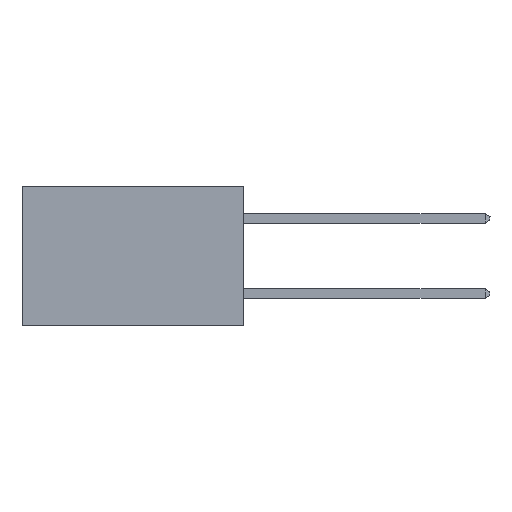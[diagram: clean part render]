
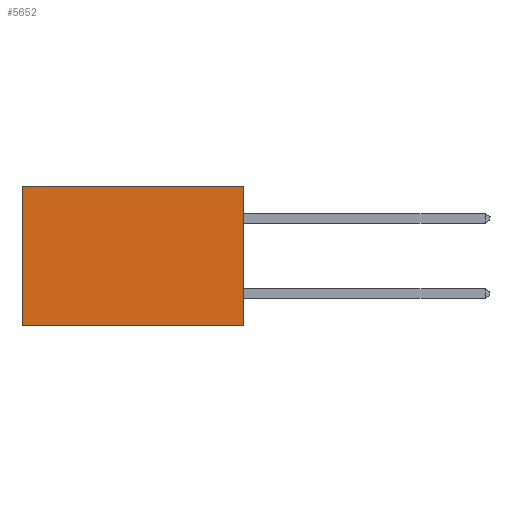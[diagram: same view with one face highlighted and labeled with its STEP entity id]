
A CAD part, left-side view. The second image highlights one B-rep face of the part: STEP entity #5652.
In plain terms, the highlighted planar face has unit normal (-1, 0, 0).
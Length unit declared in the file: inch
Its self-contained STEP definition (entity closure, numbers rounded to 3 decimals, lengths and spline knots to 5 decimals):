
#491 = VECTOR ( 'NONE', #18228, 39.37008 ) ;
#925 = ORIENTED_EDGE ( 'NONE', *, *, #9962, .F. ) ;
#2848 = EDGE_CURVE ( 'NONE', #4922, #15119, #9352, .T. ) ;
#3275 = EDGE_LOOP ( 'NONE', ( #4256, #6857, #925, #7363 ) ) ;
#4256 = ORIENTED_EDGE ( 'NONE', *, *, #2848, .T. ) ;
#4922 = VERTEX_POINT ( 'NONE', #12357 ) ;
#5003 = VECTOR ( 'NONE', #8006, 39.37008 ) ;
#5377 = VECTOR ( 'NONE', #11767, 39.37008 ) ;
#5652 = ADVANCED_FACE ( 'NONE', ( #5923 ), #5891, .F. ) ;
#5667 = CARTESIAN_POINT ( 'NONE',  ( 0.277, 0., -0.37 ) ) ;
#5861 = DIRECTION ( 'NONE',  ( 0., 0., -1. ) ) ;
#5866 = DIRECTION ( 'NONE',  ( 1., 0., 0. ) ) ;
#5891 = PLANE ( 'NONE',  #12465 ) ;
#5900 = LINE ( 'NONE', #13322, #5377 ) ;
#5923 = FACE_OUTER_BOUND ( 'NONE', #3275, .T. ) ;
#6857 = ORIENTED_EDGE ( 'NONE', *, *, #9370, .F. ) ;
#7017 = CARTESIAN_POINT ( 'NONE',  ( 0.277, 0.59, -0.37 ) ) ;
#7363 = ORIENTED_EDGE ( 'NONE', *, *, #20407, .T. ) ;
#8006 = DIRECTION ( 'NONE',  ( 0., 0., -1. ) ) ;
#8254 = DIRECTION ( 'NONE',  ( 0., 0., -1. ) ) ;
#9200 = LINE ( 'NONE', #19730, #491 ) ;
#9352 = LINE ( 'NONE', #7017, #5003 ) ;
#9370 = EDGE_CURVE ( 'NONE', #12224, #15119, #5900, .T. ) ;
#9962 = EDGE_CURVE ( 'NONE', #13469, #12224, #15740, .T. ) ;
#11767 = DIRECTION ( 'NONE',  ( 0., 1., 0. ) ) ;
#11980 = VECTOR ( 'NONE', #8254, 39.37008 ) ;
#12195 = CARTESIAN_POINT ( 'NONE',  ( 0.277, 0.59, -0.37 ) ) ;
#12224 = VERTEX_POINT ( 'NONE', #18091 ) ;
#12357 = CARTESIAN_POINT ( 'NONE',  ( 0.277, 0.59, 0. ) ) ;
#12465 = AXIS2_PLACEMENT_3D ( 'NONE', #5667, #5866, #5861 ) ;
#13322 = CARTESIAN_POINT ( 'NONE',  ( 0.277, 0., -0.37 ) ) ;
#13469 = VERTEX_POINT ( 'NONE', #20942 ) ;
#15119 = VERTEX_POINT ( 'NONE', #12195 ) ;
#15740 = LINE ( 'NONE', #16312, #11980 ) ;
#16312 = CARTESIAN_POINT ( 'NONE',  ( 0.277, 0., -0.37 ) ) ;
#18091 = CARTESIAN_POINT ( 'NONE',  ( 0.277, 0., -0.37 ) ) ;
#18228 = DIRECTION ( 'NONE',  ( 0., 1., 0. ) ) ;
#19730 = CARTESIAN_POINT ( 'NONE',  ( 0.277, 0., 0. ) ) ;
#20407 = EDGE_CURVE ( 'NONE', #13469, #4922, #9200, .T. ) ;
#20942 = CARTESIAN_POINT ( 'NONE',  ( 0.277, 0., 0. ) ) ;
